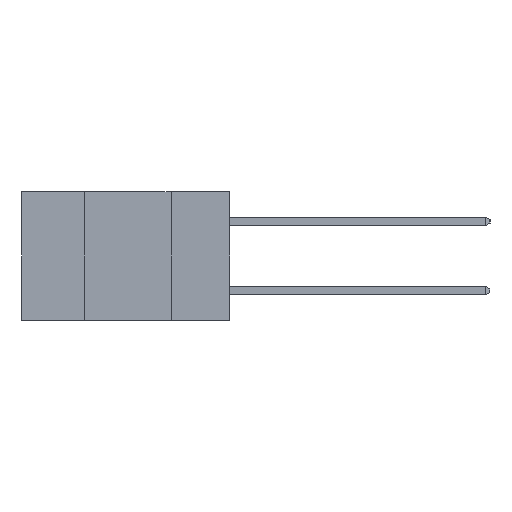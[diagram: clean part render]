
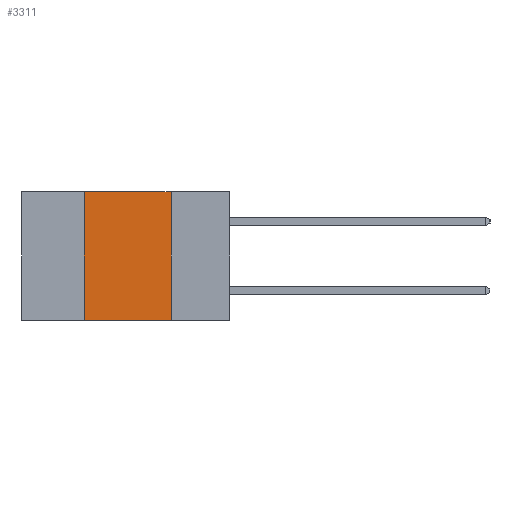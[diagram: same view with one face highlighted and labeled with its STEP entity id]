
A CAD part, left-side view. The second image highlights one B-rep face of the part: STEP entity #3311.
In plain terms, the highlighted planar face has unit normal (-1, 0, 0).
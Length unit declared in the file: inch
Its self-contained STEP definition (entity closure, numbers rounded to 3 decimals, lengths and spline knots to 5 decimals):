
#31 = DIRECTION ( 'NONE',  ( 0., -1., 0. ) ) ;
#253 = ORIENTED_EDGE ( 'NONE', *, *, #8870, .F. ) ;
#758 = LINE ( 'NONE', #5715, #16352 ) ;
#1468 = EDGE_LOOP ( 'NONE', ( #16462, #253, #3625, #10619 ) ) ;
#2881 = LINE ( 'NONE', #10483, #9412 ) ;
#3230 = CARTESIAN_POINT ( 'NONE',  ( 0., 0.17, -0.37 ) ) ;
#3311 = ADVANCED_FACE ( 'NONE', ( #4268 ), #5827, .F. ) ;
#3363 = CARTESIAN_POINT ( 'NONE',  ( 0., 0.42, 0. ) ) ;
#3625 = ORIENTED_EDGE ( 'NONE', *, *, #10178, .F. ) ;
#4268 = FACE_OUTER_BOUND ( 'NONE', #1468, .T. ) ;
#4887 = LINE ( 'NONE', #6744, #14756 ) ;
#5715 = CARTESIAN_POINT ( 'NONE',  ( 0., 0.42, 0. ) ) ;
#5827 = PLANE ( 'NONE',  #15468 ) ;
#5886 = CARTESIAN_POINT ( 'NONE',  ( 0., 0.6, 0. ) ) ;
#5959 = CARTESIAN_POINT ( 'NONE',  ( 0., 0.6, 0. ) ) ;
#6251 = EDGE_CURVE ( 'NONE', #15435, #11553, #2881, .T. ) ;
#6582 = EDGE_CURVE ( 'NONE', #6594, #11553, #4887, .T. ) ;
#6594 = VERTEX_POINT ( 'NONE', #13988 ) ;
#6744 = CARTESIAN_POINT ( 'NONE',  ( 0., 0.6, -0.37 ) ) ;
#7220 = DIRECTION ( 'NONE',  ( 0., -1., 0. ) ) ;
#8870 = EDGE_CURVE ( 'NONE', #9461, #15435, #13708, .T. ) ;
#9254 = DIRECTION ( 'NONE',  ( 0., 0., -1. ) ) ;
#9412 = VECTOR ( 'NONE', #9254, 39.37008 ) ;
#9461 = VERTEX_POINT ( 'NONE', #3363 ) ;
#10178 = EDGE_CURVE ( 'NONE', #6594, #9461, #758, .T. ) ;
#10483 = CARTESIAN_POINT ( 'NONE',  ( 0., 0.17, 0. ) ) ;
#10568 = DIRECTION ( 'NONE',  ( 1., 0., 0. ) ) ;
#10619 = ORIENTED_EDGE ( 'NONE', *, *, #6582, .T. ) ;
#11107 = DIRECTION ( 'NONE',  ( 0., 0., 1. ) ) ;
#11448 = CARTESIAN_POINT ( 'NONE',  ( 0., 0.17, 0. ) ) ;
#11553 = VERTEX_POINT ( 'NONE', #3230 ) ;
#13305 = VECTOR ( 'NONE', #7220, 39.37008 ) ;
#13708 = LINE ( 'NONE', #5959, #13305 ) ;
#13988 = CARTESIAN_POINT ( 'NONE',  ( 0., 0.42, -0.37 ) ) ;
#14756 = VECTOR ( 'NONE', #31, 39.37008 ) ;
#14815 = DIRECTION ( 'NONE',  ( 0., 0., -1. ) ) ;
#15435 = VERTEX_POINT ( 'NONE', #11448 ) ;
#15468 = AXIS2_PLACEMENT_3D ( 'NONE', #5886, #10568, #14815 ) ;
#16352 = VECTOR ( 'NONE', #11107, 39.37008 ) ;
#16462 = ORIENTED_EDGE ( 'NONE', *, *, #6251, .F. ) ;
